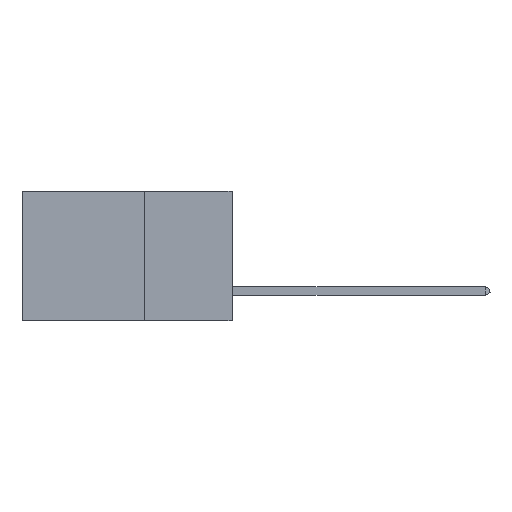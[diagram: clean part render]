
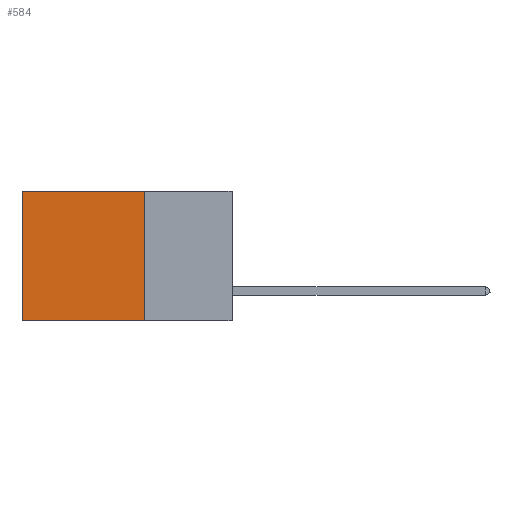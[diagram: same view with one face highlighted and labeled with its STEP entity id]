
A CAD part, left-side view. The second image highlights one B-rep face of the part: STEP entity #584.
In plain terms, the highlighted planar face has unit normal (-1, 0, 0).
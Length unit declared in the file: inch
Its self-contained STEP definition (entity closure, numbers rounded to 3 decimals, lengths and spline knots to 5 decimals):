
#584 = ADVANCED_FACE ( 'NONE', ( #8113 ), #13496, .F. ) ;
#953 = VECTOR ( 'NONE', #9366, 39.37008 ) ;
#1019 = EDGE_CURVE ( 'NONE', #20601, #20097, #4365, .T. ) ;
#2009 = DIRECTION ( 'NONE',  ( 0., 1., 0. ) ) ;
#2899 = VECTOR ( 'NONE', #2009, 39.37008 ) ;
#3254 = ORIENTED_EDGE ( 'NONE', *, *, #8966, .F. ) ;
#4365 = LINE ( 'NONE', #11834, #2899 ) ;
#5456 = LINE ( 'NONE', #19062, #14538 ) ;
#5581 = CARTESIAN_POINT ( 'NONE',  ( 0.2875, 0.6, 0. ) ) ;
#7438 = DIRECTION ( 'NONE',  ( 0., 1., 0. ) ) ;
#7509 = EDGE_LOOP ( 'NONE', ( #17049, #3254, #21941, #7868 ) ) ;
#7568 = EDGE_CURVE ( 'NONE', #20601, #23571, #18374, .T. ) ;
#7868 = ORIENTED_EDGE ( 'NONE', *, *, #1019, .T. ) ;
#7895 = CARTESIAN_POINT ( 'NONE',  ( 0.2875, 0.6, -0.37 ) ) ;
#8113 = FACE_OUTER_BOUND ( 'NONE', #7509, .T. ) ;
#8966 = EDGE_CURVE ( 'NONE', #23571, #16876, #5456, .T. ) ;
#9366 = DIRECTION ( 'NONE',  ( 0., 0., -1. ) ) ;
#9563 = LINE ( 'NONE', #5581, #15635 ) ;
#9746 = CARTESIAN_POINT ( 'NONE',  ( 0.2875, 0.25, 0. ) ) ;
#11630 = DIRECTION ( 'NONE',  ( 1., 0., 0. ) ) ;
#11834 = CARTESIAN_POINT ( 'NONE',  ( 0.2875, 0.25, 0. ) ) ;
#11863 = DIRECTION ( 'NONE',  ( 0., 0., -1. ) ) ;
#13496 = PLANE ( 'NONE',  #20403 ) ;
#14538 = VECTOR ( 'NONE', #7438, 39.37008 ) ;
#14879 = CARTESIAN_POINT ( 'NONE',  ( 0.2875, 0.25, 0. ) ) ;
#15635 = VECTOR ( 'NONE', #17063, 39.37008 ) ;
#16876 = VERTEX_POINT ( 'NONE', #7895 ) ;
#17049 = ORIENTED_EDGE ( 'NONE', *, *, #19421, .T. ) ;
#17063 = DIRECTION ( 'NONE',  ( 0., 0., -1. ) ) ;
#18374 = LINE ( 'NONE', #14879, #953 ) ;
#18448 = CARTESIAN_POINT ( 'NONE',  ( 0.2875, 0.25, -0.37 ) ) ;
#19062 = CARTESIAN_POINT ( 'NONE',  ( 0.2875, 0.25, -0.37 ) ) ;
#19421 = EDGE_CURVE ( 'NONE', #20097, #16876, #9563, .T. ) ;
#20097 = VERTEX_POINT ( 'NONE', #21995 ) ;
#20403 = AXIS2_PLACEMENT_3D ( 'NONE', #9746, #11630, #11863 ) ;
#20601 = VERTEX_POINT ( 'NONE', #22427 ) ;
#21941 = ORIENTED_EDGE ( 'NONE', *, *, #7568, .F. ) ;
#21995 = CARTESIAN_POINT ( 'NONE',  ( 0.2875, 0.6, 0. ) ) ;
#22427 = CARTESIAN_POINT ( 'NONE',  ( 0.2875, 0.25, 0. ) ) ;
#23571 = VERTEX_POINT ( 'NONE', #18448 ) ;
